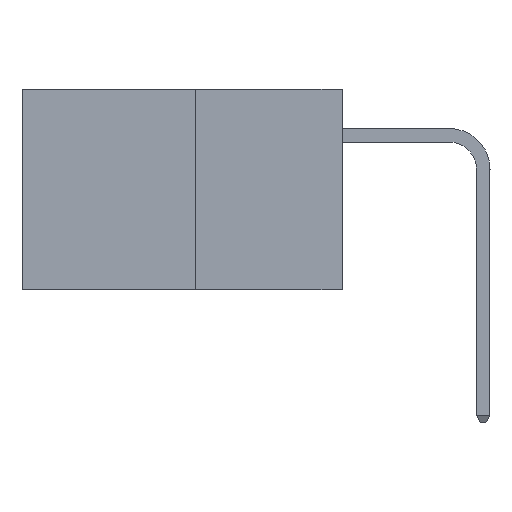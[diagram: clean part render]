
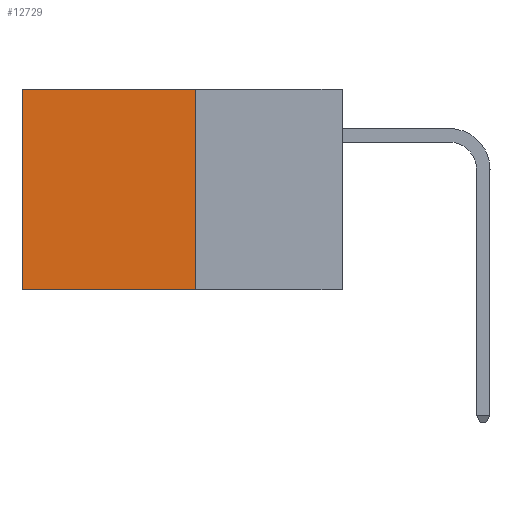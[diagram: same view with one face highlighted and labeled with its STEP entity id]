
A CAD part, left-side view. The second image highlights one B-rep face of the part: STEP entity #12729.
In plain terms, the highlighted planar face has unit normal (-1, 0, 0).
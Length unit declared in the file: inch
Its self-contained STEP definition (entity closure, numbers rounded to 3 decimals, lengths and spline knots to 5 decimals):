
#652 = ORIENTED_EDGE ( 'NONE', *, *, #12260, .T. ) ;
#1030 = VERTEX_POINT ( 'NONE', #3512 ) ;
#1253 = EDGE_CURVE ( 'NONE', #8539, #13386, #6432, .T. ) ;
#1933 = LINE ( 'NONE', #8955, #4658 ) ;
#2006 = ORIENTED_EDGE ( 'NONE', *, *, #10479, .F. ) ;
#2358 = DIRECTION ( 'NONE',  ( 0., 0., -1. ) ) ;
#2845 = EDGE_LOOP ( 'NONE', ( #652, #2006, #10376, #10677 ) ) ;
#2855 = VERTEX_POINT ( 'NONE', #11718 ) ;
#2883 = VECTOR ( 'NONE', #2358, 39.37008 ) ;
#3160 = DIRECTION ( 'NONE',  ( 0., 1., 0. ) ) ;
#3512 = CARTESIAN_POINT ( 'NONE',  ( 0.277, 0.59, 0. ) ) ;
#3615 = LINE ( 'NONE', #8140, #2883 ) ;
#4079 = VECTOR ( 'NONE', #6197, 39.37008 ) ;
#4415 = PLANE ( 'NONE',  #9836 ) ;
#4467 = DIRECTION ( 'NONE',  ( 0., 0., -1. ) ) ;
#4514 = CARTESIAN_POINT ( 'NONE',  ( 0.277, 0.27, -0.37 ) ) ;
#4581 = EDGE_CURVE ( 'NONE', #8539, #1030, #8867, .T. ) ;
#4658 = VECTOR ( 'NONE', #3160, 39.37008 ) ;
#5434 = VECTOR ( 'NONE', #9130, 39.37008 ) ;
#6197 = DIRECTION ( 'NONE',  ( 0., 0., -1. ) ) ;
#6432 = LINE ( 'NONE', #11365, #4079 ) ;
#8140 = CARTESIAN_POINT ( 'NONE',  ( 0.277, 0.59, -0.37 ) ) ;
#8539 = VERTEX_POINT ( 'NONE', #14881 ) ;
#8867 = LINE ( 'NONE', #14971, #5434 ) ;
#8955 = CARTESIAN_POINT ( 'NONE',  ( 0.277, 0.27, -0.37 ) ) ;
#9111 = CARTESIAN_POINT ( 'NONE',  ( 0.277, 0.27, -0.37 ) ) ;
#9130 = DIRECTION ( 'NONE',  ( 0., 1., 0. ) ) ;
#9836 = AXIS2_PLACEMENT_3D ( 'NONE', #9111, #11473, #4467 ) ;
#10376 = ORIENTED_EDGE ( 'NONE', *, *, #1253, .F. ) ;
#10479 = EDGE_CURVE ( 'NONE', #13386, #2855, #1933, .T. ) ;
#10677 = ORIENTED_EDGE ( 'NONE', *, *, #4581, .T. ) ;
#11365 = CARTESIAN_POINT ( 'NONE',  ( 0.277, 0.27, -0.37 ) ) ;
#11473 = DIRECTION ( 'NONE',  ( 1., 0., 0. ) ) ;
#11718 = CARTESIAN_POINT ( 'NONE',  ( 0.277, 0.59, -0.37 ) ) ;
#12260 = EDGE_CURVE ( 'NONE', #1030, #2855, #3615, .T. ) ;
#12729 = ADVANCED_FACE ( 'NONE', ( #14915 ), #4415, .F. ) ;
#13386 = VERTEX_POINT ( 'NONE', #4514 ) ;
#14881 = CARTESIAN_POINT ( 'NONE',  ( 0.277, 0.27, 0. ) ) ;
#14915 = FACE_OUTER_BOUND ( 'NONE', #2845, .T. ) ;
#14971 = CARTESIAN_POINT ( 'NONE',  ( 0.277, 0.27, 0. ) ) ;
